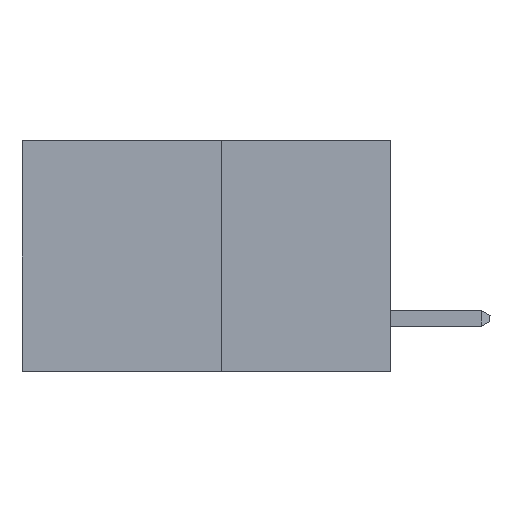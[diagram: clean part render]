
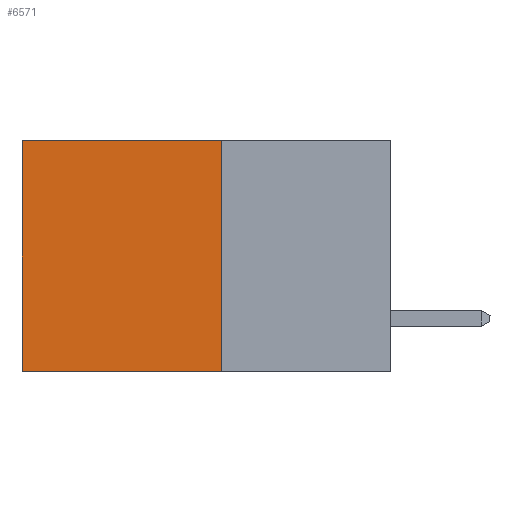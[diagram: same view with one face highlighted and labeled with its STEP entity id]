
A CAD part, left-side view. The second image highlights one B-rep face of the part: STEP entity #6571.
In plain terms, the highlighted planar face has unit normal (-1, 0, 0).
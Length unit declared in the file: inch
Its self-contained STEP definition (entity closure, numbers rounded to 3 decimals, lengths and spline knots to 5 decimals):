
#501 = ORIENTED_EDGE ( 'NONE', *, *, #9752, .F. ) ;
#700 = AXIS2_PLACEMENT_3D ( 'NONE', #3358, #3348, #3345 ) ;
#1287 = VERTEX_POINT ( 'NONE', #7530 ) ;
#1667 = LINE ( 'NONE', #5677, #5736 ) ;
#2537 = CARTESIAN_POINT ( 'NONE',  ( 0.277, 0.59, -0.37 ) ) ;
#2621 = LINE ( 'NONE', #4456, #5051 ) ;
#3345 = DIRECTION ( 'NONE',  ( 0., 0., -1. ) ) ;
#3348 = DIRECTION ( 'NONE',  ( 1., 0., 0. ) ) ;
#3358 = CARTESIAN_POINT ( 'NONE',  ( 0.277, 0.27, -0.37 ) ) ;
#3385 = PLANE ( 'NONE',  #700 ) ;
#4323 = EDGE_CURVE ( 'NONE', #6035, #1287, #2621, .T. ) ;
#4456 = CARTESIAN_POINT ( 'NONE',  ( 0.277, 0.27, 0. ) ) ;
#4490 = VERTEX_POINT ( 'NONE', #9932 ) ;
#4665 = DIRECTION ( 'NONE',  ( 0., 1., 0. ) ) ;
#5051 = VECTOR ( 'NONE', #7942, 39.37008 ) ;
#5392 = DIRECTION ( 'NONE',  ( 0., 0., -1. ) ) ;
#5450 = VECTOR ( 'NONE', #5392, 39.37008 ) ;
#5579 = FACE_OUTER_BOUND ( 'NONE', #5790, .T. ) ;
#5610 = DIRECTION ( 'NONE',  ( 0., 0., -1. ) ) ;
#5677 = CARTESIAN_POINT ( 'NONE',  ( 0.277, 0.59, -0.37 ) ) ;
#5715 = VECTOR ( 'NONE', #4665, 39.37008 ) ;
#5736 = VECTOR ( 'NONE', #5610, 39.37008 ) ;
#5790 = EDGE_LOOP ( 'NONE', ( #7303, #5972, #501, #9734 ) ) ;
#5972 = ORIENTED_EDGE ( 'NONE', *, *, #8599, .F. ) ;
#6035 = VERTEX_POINT ( 'NONE', #7011 ) ;
#6152 = CARTESIAN_POINT ( 'NONE',  ( 0.277, 0.27, -0.37 ) ) ;
#6571 = ADVANCED_FACE ( 'NONE', ( #5579 ), #3385, .F. ) ;
#6662 = VERTEX_POINT ( 'NONE', #2537 ) ;
#7011 = CARTESIAN_POINT ( 'NONE',  ( 0.277, 0.27, 0. ) ) ;
#7303 = ORIENTED_EDGE ( 'NONE', *, *, #7781, .T. ) ;
#7530 = CARTESIAN_POINT ( 'NONE',  ( 0.277, 0.59, 0. ) ) ;
#7739 = LINE ( 'NONE', #6152, #5450 ) ;
#7781 = EDGE_CURVE ( 'NONE', #1287, #6662, #1667, .T. ) ;
#7942 = DIRECTION ( 'NONE',  ( 0., 1., 0. ) ) ;
#8599 = EDGE_CURVE ( 'NONE', #4490, #6662, #9810, .T. ) ;
#9087 = CARTESIAN_POINT ( 'NONE',  ( 0.277, 0.27, -0.37 ) ) ;
#9734 = ORIENTED_EDGE ( 'NONE', *, *, #4323, .T. ) ;
#9752 = EDGE_CURVE ( 'NONE', #6035, #4490, #7739, .T. ) ;
#9810 = LINE ( 'NONE', #9087, #5715 ) ;
#9932 = CARTESIAN_POINT ( 'NONE',  ( 0.277, 0.27, -0.37 ) ) ;
